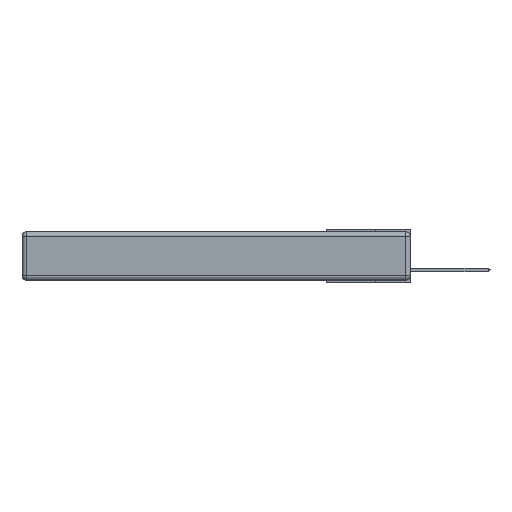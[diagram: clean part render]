
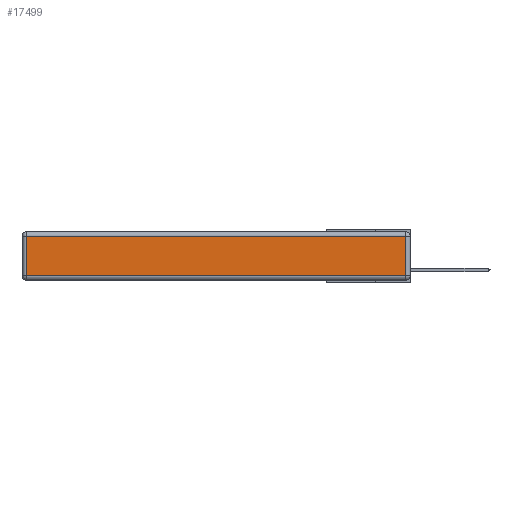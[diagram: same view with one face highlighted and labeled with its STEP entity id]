
A CAD part, left-side view. The second image highlights one B-rep face of the part: STEP entity #17499.
In plain terms, the highlighted planar face has unit normal (-1, 0, 0).
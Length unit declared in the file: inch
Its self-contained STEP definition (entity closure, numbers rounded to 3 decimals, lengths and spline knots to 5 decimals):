
#648 = EDGE_CURVE ( 'NONE', #15848, #9124, #19278, .T. ) ;
#3871 = LINE ( 'NONE', #33735, #32235 ) ;
#5350 = VERTEX_POINT ( 'NONE', #18388 ) ;
#6125 = CARTESIAN_POINT ( 'NONE',  ( 0., 0.03, -0.343 ) ) ;
#6214 = ORIENTED_EDGE ( 'NONE', *, *, #11869, .T. ) ;
#6465 = DIRECTION ( 'NONE',  ( 0., 0., 1. ) ) ;
#9070 = LINE ( 'NONE', #6125, #14381 ) ;
#9124 = VERTEX_POINT ( 'NONE', #24242 ) ;
#10503 = CARTESIAN_POINT ( 'NONE',  ( 0., 2.72, -0.313 ) ) ;
#10677 = ORIENTED_EDGE ( 'NONE', *, *, #30723, .T. ) ;
#11869 = EDGE_CURVE ( 'NONE', #9124, #16303, #9070, .T. ) ;
#12689 = CARTESIAN_POINT ( 'NONE',  ( 0., 2.72, -0.343 ) ) ;
#13088 = EDGE_CURVE ( 'NONE', #5350, #15848, #27460, .T. ) ;
#14319 = VECTOR ( 'NONE', #32752, 39.37008 ) ;
#14381 = VECTOR ( 'NONE', #6465, 39.37008 ) ;
#14729 = VECTOR ( 'NONE', #26142, 39.37008 ) ;
#15848 = VERTEX_POINT ( 'NONE', #10503 ) ;
#16303 = VERTEX_POINT ( 'NONE', #33602 ) ;
#16469 = CARTESIAN_POINT ( 'NONE',  ( 0., 0., -0.313 ) ) ;
#16912 = DIRECTION ( 'NONE',  ( 0., 0., 1. ) ) ;
#17499 = ADVANCED_FACE ( 'NONE', ( #27823 ), #25071, .T. ) ;
#18388 = CARTESIAN_POINT ( 'NONE',  ( 0., 2.72, -0.03 ) ) ;
#18853 = DIRECTION ( 'NONE',  ( -1., 0., 0. ) ) ;
#19278 = LINE ( 'NONE', #16469, #14319 ) ;
#20782 = DIRECTION ( 'NONE',  ( 0., 1., 0. ) ) ;
#22982 = ORIENTED_EDGE ( 'NONE', *, *, #13088, .T. ) ;
#24164 = CARTESIAN_POINT ( 'NONE',  ( 0., 0., -0.343 ) ) ;
#24242 = CARTESIAN_POINT ( 'NONE',  ( 0., 0.03, -0.313 ) ) ;
#25071 = PLANE ( 'NONE',  #25501 ) ;
#25501 = AXIS2_PLACEMENT_3D ( 'NONE', #24164, #18853, #16912 ) ;
#26142 = DIRECTION ( 'NONE',  ( 0., 0., -1. ) ) ;
#27460 = LINE ( 'NONE', #12689, #14729 ) ;
#27823 = FACE_OUTER_BOUND ( 'NONE', #31127, .T. ) ;
#30723 = EDGE_CURVE ( 'NONE', #16303, #5350, #3871, .T. ) ;
#31127 = EDGE_LOOP ( 'NONE', ( #32786, #6214, #10677, #22982 ) ) ;
#32235 = VECTOR ( 'NONE', #20782, 39.37008 ) ;
#32752 = DIRECTION ( 'NONE',  ( 0., -1., 0. ) ) ;
#32786 = ORIENTED_EDGE ( 'NONE', *, *, #648, .T. ) ;
#33602 = CARTESIAN_POINT ( 'NONE',  ( 0., 0.03, -0.03 ) ) ;
#33735 = CARTESIAN_POINT ( 'NONE',  ( 0., 2.75, -0.03 ) ) ;
